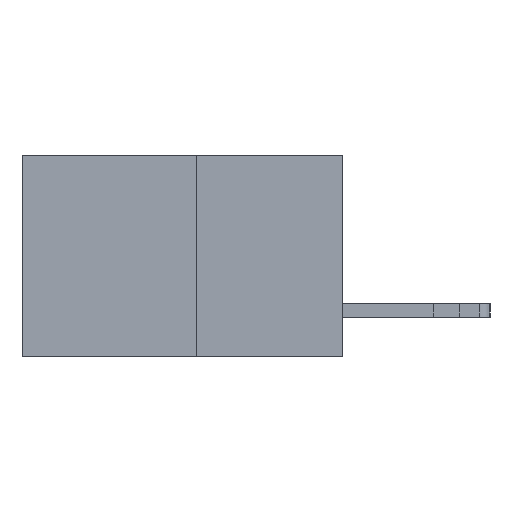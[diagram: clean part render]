
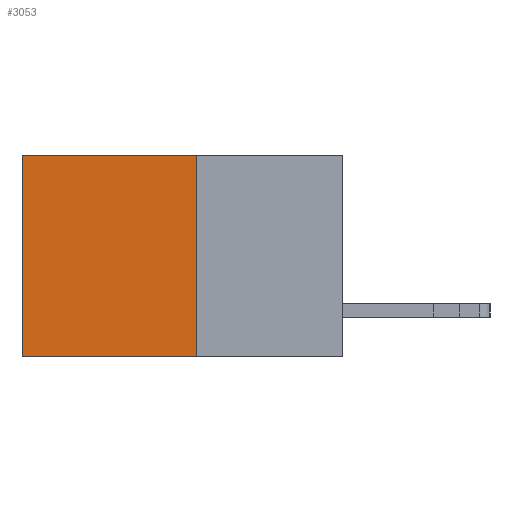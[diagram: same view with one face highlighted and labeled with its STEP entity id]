
A CAD part, left-side view. The second image highlights one B-rep face of the part: STEP entity #3053.
In plain terms, the highlighted planar face has unit normal (-1, 0, 0).
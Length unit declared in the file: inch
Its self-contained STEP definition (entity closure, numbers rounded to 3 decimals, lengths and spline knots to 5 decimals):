
#239 = CARTESIAN_POINT ( 'NONE',  ( 0.277, 0.27, -0.37 ) ) ;
#735 = LINE ( 'NONE', #17438, #8104 ) ;
#1125 = ORIENTED_EDGE ( 'NONE', *, *, #1379, .T. ) ;
#1379 = EDGE_CURVE ( 'NONE', #13918, #9612, #735, .T. ) ;
#1578 = CARTESIAN_POINT ( 'NONE',  ( 0.277, 0.27, 0. ) ) ;
#1674 = EDGE_CURVE ( 'NONE', #9612, #11086, #13780, .T. ) ;
#2429 = VECTOR ( 'NONE', #10988, 39.37008 ) ;
#2457 = VECTOR ( 'NONE', #4002, 39.37008 ) ;
#2696 = VECTOR ( 'NONE', #6287, 39.37008 ) ;
#3053 = ADVANCED_FACE ( 'NONE', ( #7883 ), #4236, .F. ) ;
#3802 = ORIENTED_EDGE ( 'NONE', *, *, #17760, .F. ) ;
#3813 = CARTESIAN_POINT ( 'NONE',  ( 0.277, 0.59, -0.37 ) ) ;
#3895 = DIRECTION ( 'NONE',  ( 0., 0., -1. ) ) ;
#3920 = DIRECTION ( 'NONE',  ( 1., 0., 0. ) ) ;
#3961 = CARTESIAN_POINT ( 'NONE',  ( 0.277, 0.27, -0.37 ) ) ;
#4002 = DIRECTION ( 'NONE',  ( 0., 0., -1. ) ) ;
#4100 = CARTESIAN_POINT ( 'NONE',  ( 0.277, 0.59, 0. ) ) ;
#4236 = PLANE ( 'NONE',  #8747 ) ;
#4931 = CARTESIAN_POINT ( 'NONE',  ( 0.277, 0.27, -0.37 ) ) ;
#5165 = EDGE_CURVE ( 'NONE', #13918, #9941, #14184, .T. ) ;
#6287 = DIRECTION ( 'NONE',  ( 0., 1., 0. ) ) ;
#7883 = FACE_OUTER_BOUND ( 'NONE', #14423, .T. ) ;
#8104 = VECTOR ( 'NONE', #17762, 39.37008 ) ;
#8747 = AXIS2_PLACEMENT_3D ( 'NONE', #3961, #3920, #3895 ) ;
#9612 = VERTEX_POINT ( 'NONE', #4100 ) ;
#9941 = VERTEX_POINT ( 'NONE', #239 ) ;
#10898 = CARTESIAN_POINT ( 'NONE',  ( 0.277, 0.27, -0.37 ) ) ;
#10988 = DIRECTION ( 'NONE',  ( 0., 0., -1. ) ) ;
#11086 = VERTEX_POINT ( 'NONE', #15627 ) ;
#13481 = ORIENTED_EDGE ( 'NONE', *, *, #5165, .F. ) ;
#13610 = ORIENTED_EDGE ( 'NONE', *, *, #1674, .T. ) ;
#13780 = LINE ( 'NONE', #3813, #2457 ) ;
#13918 = VERTEX_POINT ( 'NONE', #1578 ) ;
#14184 = LINE ( 'NONE', #10898, #2429 ) ;
#14423 = EDGE_LOOP ( 'NONE', ( #13610, #3802, #13481, #1125 ) ) ;
#15627 = CARTESIAN_POINT ( 'NONE',  ( 0.277, 0.59, -0.37 ) ) ;
#17223 = LINE ( 'NONE', #4931, #2696 ) ;
#17438 = CARTESIAN_POINT ( 'NONE',  ( 0.277, 0.27, 0. ) ) ;
#17760 = EDGE_CURVE ( 'NONE', #9941, #11086, #17223, .T. ) ;
#17762 = DIRECTION ( 'NONE',  ( 0., 1., 0. ) ) ;
